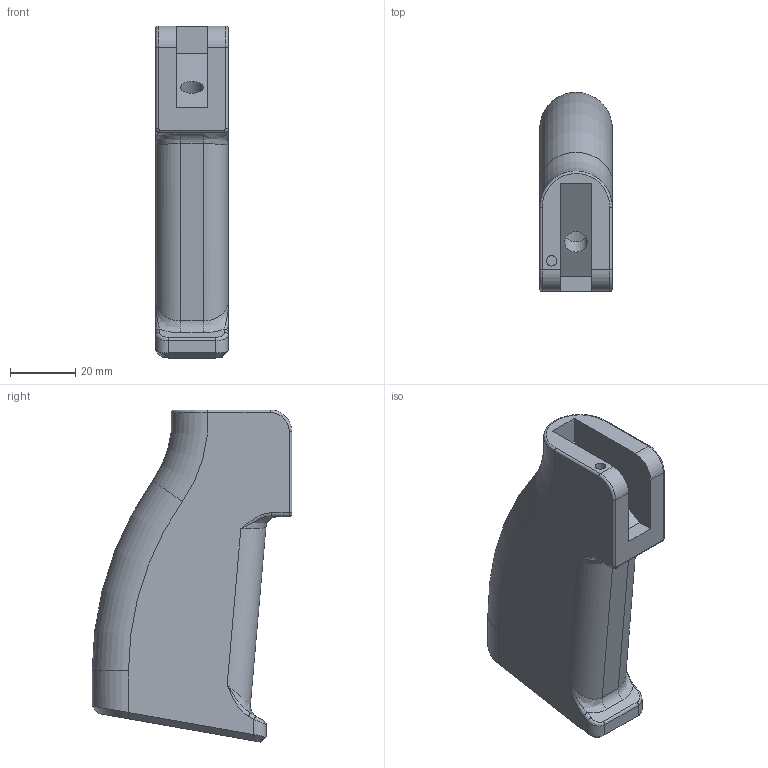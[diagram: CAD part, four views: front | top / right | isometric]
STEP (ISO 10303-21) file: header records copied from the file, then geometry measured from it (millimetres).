
FILE_DESCRIPTION(/* description */ (''),/* implementation_level */ '2;1');
FILE_NAME(/* name */ 'SG22 Pistol Grip Release.step',/* time_stamp */ '2021-03-18T08:57:11-06:00',/* author */ (''),/* organization */ (''),/* preprocessor_version */ 'ST-DEVELOPER v18.1',/* originating_system */ 'Autodesk Translation Framework v9.10.0.1330',/* authorisation */ '');
FILE_SCHEMA (('AUTOMOTIVE_DESIGN { 1 0 10303 214 3 1 1 }'));
Length unit declared in the file: millimetre
Products named in the file (1): Brace V2
Bounding box: 22.23 x 61.09 x 101.66 mm (x, y, z)
Volume: 53580.8 mm3; surface area: 21541.6 mm2
Topology: 1 solids, 1 shells, 69 faces, 168 edges, 99 vertices
Faces by surface type: cylinder 23, plane 21, bspline 20, torus 5
Full cylindrical faces by diameter (mm): 3.175 x1, 7.163 x1
Entity records: 3017 total; most frequent: CARTESIAN_POINT 1422, ORIENTED_EDGE 328, DIRECTION 306, EDGE_CURVE 164, AXIS2_PLACEMENT_3D 112, VERTEX_POINT 99, LINE 82, VECTOR 82
